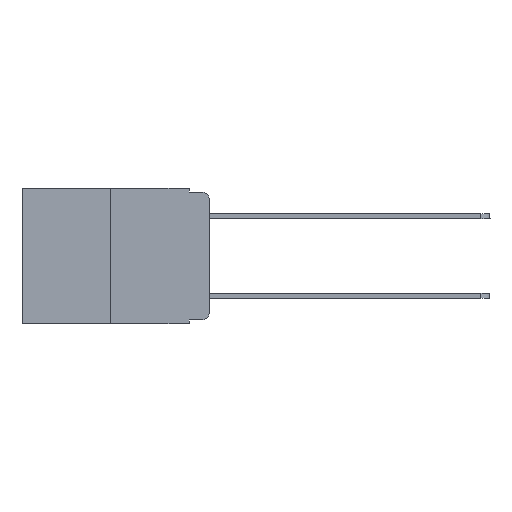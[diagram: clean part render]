
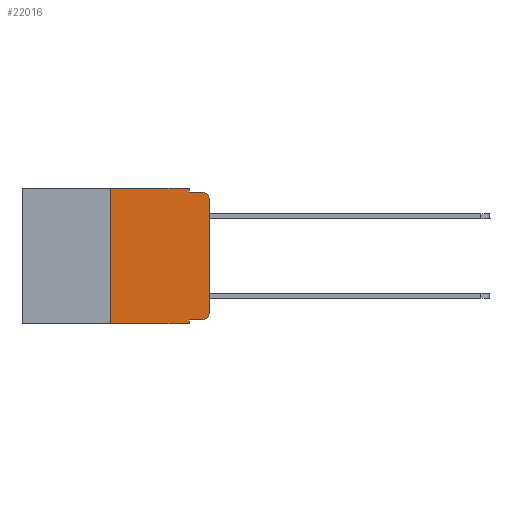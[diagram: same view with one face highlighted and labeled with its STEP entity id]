
A CAD part, left-side view. The second image highlights one B-rep face of the part: STEP entity #22016.
In plain terms, the highlighted planar face has unit normal (-1, 0, 0).
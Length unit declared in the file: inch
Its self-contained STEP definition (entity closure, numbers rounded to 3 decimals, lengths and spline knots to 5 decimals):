
#72 = DIRECTION ( 'NONE',  ( 0., 0., 1. ) ) ;
#181 = VERTEX_POINT ( 'NONE', #14170 ) ;
#530 = EDGE_CURVE ( 'NONE', #9012, #11138, #5819, .T. ) ;
#829 = VECTOR ( 'NONE', #20951, 39.37008 ) ;
#1042 = CARTESIAN_POINT ( 'NONE',  ( 0., 0.473, -0.343 ) ) ;
#1844 = EDGE_CURVE ( 'NONE', #19509, #5484, #17784, .T. ) ;
#2167 = LINE ( 'NONE', #17419, #8565 ) ;
#2203 = CARTESIAN_POINT ( 'NONE',  ( 0., 0.473, 0. ) ) ;
#2806 = DIRECTION ( 'NONE',  ( 1., 0., 0. ) ) ;
#3100 = VECTOR ( 'NONE', #20779, 39.37008 ) ;
#3291 = CARTESIAN_POINT ( 'NONE',  ( 0., 0.473, 0. ) ) ;
#3653 = DIRECTION ( 'NONE',  ( -1., 0., 0. ) ) ;
#3685 = ORIENTED_EDGE ( 'NONE', *, *, #20433, .T. ) ;
#3828 = VERTEX_POINT ( 'NONE', #20181 ) ;
#4051 = LINE ( 'NONE', #1042, #14054 ) ;
#4871 = DIRECTION ( 'NONE',  ( 0., 0., 1. ) ) ;
#4926 = EDGE_CURVE ( 'NONE', #20866, #9012, #2167, .T. ) ;
#5153 = VERTEX_POINT ( 'NONE', #17880 ) ;
#5484 = VERTEX_POINT ( 'NONE', #9176 ) ;
#5539 = CIRCLE ( 'NONE', #24230, 0.02 ) ;
#5620 = EDGE_CURVE ( 'NONE', #3828, #5153, #10889, .T. ) ;
#5819 = LINE ( 'NONE', #8783, #8424 ) ;
#6405 = CARTESIAN_POINT ( 'NONE',  ( 0., 0.051, 0. ) ) ;
#6503 = DIRECTION ( 'NONE',  ( 0., 0., -1. ) ) ;
#6569 = LINE ( 'NONE', #6405, #3100 ) ;
#6656 = DIRECTION ( 'NONE',  ( -1., 0., 0. ) ) ;
#6804 = CARTESIAN_POINT ( 'NONE',  ( 0., 0., 0. ) ) ;
#7015 = FACE_OUTER_BOUND ( 'NONE', #19416, .T. ) ;
#7628 = VECTOR ( 'NONE', #72, 39.37008 ) ;
#7674 = CARTESIAN_POINT ( 'NONE',  ( 0., 0.051, -0.333 ) ) ;
#7719 = ORIENTED_EDGE ( 'NONE', *, *, #20374, .T. ) ;
#8424 = VECTOR ( 'NONE', #10371, 39.37008 ) ;
#8438 = CIRCLE ( 'NONE', #20078, 0.02 ) ;
#8565 = VECTOR ( 'NONE', #13475, 39.37008 ) ;
#8783 = CARTESIAN_POINT ( 'NONE',  ( 0., 0.051, -0.01 ) ) ;
#9012 = VERTEX_POINT ( 'NONE', #12506 ) ;
#9176 = CARTESIAN_POINT ( 'NONE',  ( 0., 0.02, -0.333 ) ) ;
#9449 = ORIENTED_EDGE ( 'NONE', *, *, #1844, .T. ) ;
#10371 = DIRECTION ( 'NONE',  ( 0., -1., 0. ) ) ;
#10857 = DIRECTION ( 'NONE',  ( 0., 0., -1. ) ) ;
#10889 = LINE ( 'NONE', #16836, #7628 ) ;
#11138 = VERTEX_POINT ( 'NONE', #23119 ) ;
#11305 = CARTESIAN_POINT ( 'NONE',  ( 0., 0.051, -0.333 ) ) ;
#11747 = CARTESIAN_POINT ( 'NONE',  ( 0., 0.051, 0. ) ) ;
#12345 = VECTOR ( 'NONE', #4871, 39.37008 ) ;
#12401 = VERTEX_POINT ( 'NONE', #16911 ) ;
#12506 = CARTESIAN_POINT ( 'NONE',  ( 0., 0.051, -0.01 ) ) ;
#12648 = ORIENTED_EDGE ( 'NONE', *, *, #22755, .F. ) ;
#13475 = DIRECTION ( 'NONE',  ( 0., 0., -1. ) ) ;
#14053 = DIRECTION ( 'NONE',  ( 0., -1., 0. ) ) ;
#14054 = VECTOR ( 'NONE', #14053, 39.37008 ) ;
#14170 = CARTESIAN_POINT ( 'NONE',  ( 0., 0.051, -0.343 ) ) ;
#15363 = DIRECTION ( 'NONE',  ( 0., -1., 0. ) ) ;
#15759 = VERTEX_POINT ( 'NONE', #20168 ) ;
#16708 = EDGE_CURVE ( 'NONE', #19509, #181, #6569, .T. ) ;
#16836 = CARTESIAN_POINT ( 'NONE',  ( 0., 0.25, 0. ) ) ;
#16837 = DIRECTION ( 'NONE',  ( 0., 0., -1. ) ) ;
#16911 = CARTESIAN_POINT ( 'NONE',  ( 0., 0., -0.03 ) ) ;
#16950 = AXIS2_PLACEMENT_3D ( 'NONE', #3291, #2806, #10857 ) ;
#17200 = ORIENTED_EDGE ( 'NONE', *, *, #530, .F. ) ;
#17316 = LINE ( 'NONE', #6804, #12345 ) ;
#17419 = CARTESIAN_POINT ( 'NONE',  ( 0., 0.051, 0. ) ) ;
#17784 = LINE ( 'NONE', #7674, #829 ) ;
#17880 = CARTESIAN_POINT ( 'NONE',  ( 0., 0.25, 0. ) ) ;
#17909 = CARTESIAN_POINT ( 'NONE',  ( 0., 0.02, -0.03 ) ) ;
#19306 = EDGE_CURVE ( 'NONE', #12401, #11138, #8438, .T. ) ;
#19318 = VECTOR ( 'NONE', #15363, 39.37008 ) ;
#19372 = ORIENTED_EDGE ( 'NONE', *, *, #5620, .F. ) ;
#19416 = EDGE_LOOP ( 'NONE', ( #7719, #22131, #17200, #19468, #12648, #19372, #3685, #21393, #9449, #22757 ) ) ;
#19468 = ORIENTED_EDGE ( 'NONE', *, *, #4926, .F. ) ;
#19509 = VERTEX_POINT ( 'NONE', #11305 ) ;
#20078 = AXIS2_PLACEMENT_3D ( 'NONE', #17909, #6656, #6503 ) ;
#20168 = CARTESIAN_POINT ( 'NONE',  ( 0., 0., -0.313 ) ) ;
#20181 = CARTESIAN_POINT ( 'NONE',  ( 0., 0.25, -0.343 ) ) ;
#20374 = EDGE_CURVE ( 'NONE', #15759, #12401, #17316, .T. ) ;
#20433 = EDGE_CURVE ( 'NONE', #3828, #181, #4051, .T. ) ;
#20470 = CARTESIAN_POINT ( 'NONE',  ( 0., 0.02, -0.313 ) ) ;
#20779 = DIRECTION ( 'NONE',  ( 0., 0., -1. ) ) ;
#20790 = LINE ( 'NONE', #2203, #19318 ) ;
#20866 = VERTEX_POINT ( 'NONE', #11747 ) ;
#20951 = DIRECTION ( 'NONE',  ( 0., -1., 0. ) ) ;
#21393 = ORIENTED_EDGE ( 'NONE', *, *, #16708, .F. ) ;
#22016 = ADVANCED_FACE ( 'NONE', ( #7015 ), #23399, .F. ) ;
#22131 = ORIENTED_EDGE ( 'NONE', *, *, #19306, .T. ) ;
#22583 = EDGE_CURVE ( 'NONE', #5484, #15759, #5539, .T. ) ;
#22755 = EDGE_CURVE ( 'NONE', #5153, #20866, #20790, .T. ) ;
#22757 = ORIENTED_EDGE ( 'NONE', *, *, #22583, .T. ) ;
#23119 = CARTESIAN_POINT ( 'NONE',  ( 0., 0.02, -0.01 ) ) ;
#23399 = PLANE ( 'NONE',  #16950 ) ;
#24230 = AXIS2_PLACEMENT_3D ( 'NONE', #20470, #3653, #16837 ) ;
